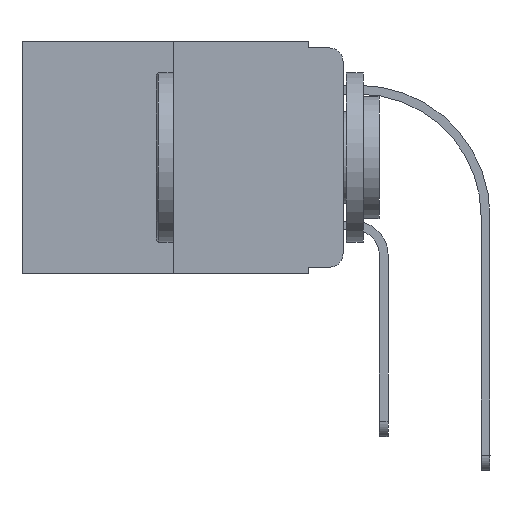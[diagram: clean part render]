
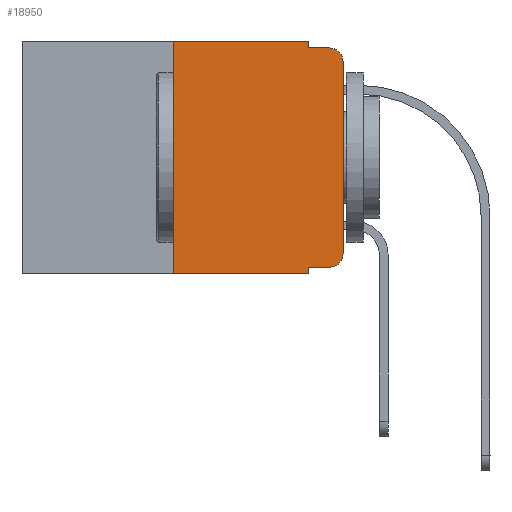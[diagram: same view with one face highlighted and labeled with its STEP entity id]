
A CAD part, left-side view. The second image highlights one B-rep face of the part: STEP entity #18950.
In plain terms, the highlighted planar face has unit normal (-1, 0, 0).
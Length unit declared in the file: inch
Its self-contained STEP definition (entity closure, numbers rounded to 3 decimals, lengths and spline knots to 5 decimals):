
#27 = AXIS2_PLACEMENT_3D ( 'NONE', #23478, #3004, #5293 ) ;
#212 = CARTESIAN_POINT ( 'NONE',  ( 0., 0.02, -0.03 ) ) ;
#581 = VERTEX_POINT ( 'NONE', #647 ) ;
#594 = CIRCLE ( 'NONE', #23664, 0.02 ) ;
#647 = CARTESIAN_POINT ( 'NONE',  ( 0., 0.25, -0.343 ) ) ;
#658 = LINE ( 'NONE', #11733, #10816 ) ;
#1832 = EDGE_CURVE ( 'NONE', #17735, #10853, #594, .T. ) ;
#1859 = ORIENTED_EDGE ( 'NONE', *, *, #13389, .F. ) ;
#2103 = ORIENTED_EDGE ( 'NONE', *, *, #11998, .F. ) ;
#2386 = CARTESIAN_POINT ( 'NONE',  ( 0., 0.051, 0. ) ) ;
#2435 = CARTESIAN_POINT ( 'NONE',  ( 0., 0.02, -0.313 ) ) ;
#2804 = DIRECTION ( 'NONE',  ( 0., -1., 0. ) ) ;
#3004 = DIRECTION ( 'NONE',  ( 1., 0., 0. ) ) ;
#3127 = LINE ( 'NONE', #14115, #8540 ) ;
#4176 = VERTEX_POINT ( 'NONE', #21479 ) ;
#4215 = LINE ( 'NONE', #22547, #14150 ) ;
#4911 = CARTESIAN_POINT ( 'NONE',  ( 0., 0.051, -0.333 ) ) ;
#5267 = CARTESIAN_POINT ( 'NONE',  ( 0., 0.051, -0.333 ) ) ;
#5293 = DIRECTION ( 'NONE',  ( 0., 0., -1. ) ) ;
#5890 = DIRECTION ( 'NONE',  ( 0., 0., -1. ) ) ;
#5921 = DIRECTION ( 'NONE',  ( 0., -1., 0. ) ) ;
#5958 = VERTEX_POINT ( 'NONE', #13751 ) ;
#6118 = ORIENTED_EDGE ( 'NONE', *, *, #1832, .T. ) ;
#7302 = DIRECTION ( 'NONE',  ( 0., 0., -1. ) ) ;
#7472 = ORIENTED_EDGE ( 'NONE', *, *, #21072, .T. ) ;
#7590 = DIRECTION ( 'NONE',  ( 0., 0., 1. ) ) ;
#8540 = VECTOR ( 'NONE', #16400, 39.37008 ) ;
#8892 = VECTOR ( 'NONE', #2804, 39.37008 ) ;
#10391 = EDGE_CURVE ( 'NONE', #581, #14768, #11678, .T. ) ;
#10418 = EDGE_LOOP ( 'NONE', ( #20623, #7472, #2103, #12338, #1859, #22718, #11884, #15980, #13289, #6118 ) ) ;
#10816 = VECTOR ( 'NONE', #17046, 39.37008 ) ;
#10853 = VERTEX_POINT ( 'NONE', #14607 ) ;
#10857 = AXIS2_PLACEMENT_3D ( 'NONE', #212, #20437, #19238 ) ;
#11126 = VERTEX_POINT ( 'NONE', #19862 ) ;
#11250 = CIRCLE ( 'NONE', #10857, 0.02 ) ;
#11678 = LINE ( 'NONE', #22404, #20807 ) ;
#11733 = CARTESIAN_POINT ( 'NONE',  ( 0., 0., 0. ) ) ;
#11884 = ORIENTED_EDGE ( 'NONE', *, *, #20402, .T. ) ;
#11998 = EDGE_CURVE ( 'NONE', #5958, #20988, #12323, .T. ) ;
#12323 = LINE ( 'NONE', #21846, #22447 ) ;
#12338 = ORIENTED_EDGE ( 'NONE', *, *, #15629, .F. ) ;
#12534 = PLANE ( 'NONE',  #27 ) ;
#12624 = DIRECTION ( 'NONE',  ( -1., 0., 0. ) ) ;
#13283 = VERTEX_POINT ( 'NONE', #20157 ) ;
#13289 = ORIENTED_EDGE ( 'NONE', *, *, #19172, .T. ) ;
#13389 = EDGE_CURVE ( 'NONE', #14768, #13283, #4215, .T. ) ;
#13458 = CARTESIAN_POINT ( 'NONE',  ( 0., 0.02, -0.333 ) ) ;
#13751 = CARTESIAN_POINT ( 'NONE',  ( 0., 0.051, -0.01 ) ) ;
#14115 = CARTESIAN_POINT ( 'NONE',  ( 0., 0.051, 0. ) ) ;
#14150 = VECTOR ( 'NONE', #5921, 39.37008 ) ;
#14607 = CARTESIAN_POINT ( 'NONE',  ( 0., 0., -0.313 ) ) ;
#14768 = VERTEX_POINT ( 'NONE', #23671 ) ;
#15044 = LINE ( 'NONE', #5267, #23093 ) ;
#15134 = VECTOR ( 'NONE', #5890, 39.37008 ) ;
#15629 = EDGE_CURVE ( 'NONE', #13283, #5958, #3127, .T. ) ;
#15980 = ORIENTED_EDGE ( 'NONE', *, *, #22397, .F. ) ;
#16064 = LINE ( 'NONE', #23400, #8892 ) ;
#16400 = DIRECTION ( 'NONE',  ( 0., 0., -1. ) ) ;
#17046 = DIRECTION ( 'NONE',  ( 0., 0., 1. ) ) ;
#17735 = VERTEX_POINT ( 'NONE', #13458 ) ;
#18950 = ADVANCED_FACE ( 'NONE', ( #22894 ), #12534, .F. ) ;
#19172 = EDGE_CURVE ( 'NONE', #19557, #17735, #15044, .T. ) ;
#19238 = DIRECTION ( 'NONE',  ( 0., 0., -1. ) ) ;
#19557 = VERTEX_POINT ( 'NONE', #4911 ) ;
#19674 = DIRECTION ( 'NONE',  ( 0., -1., 0. ) ) ;
#19862 = CARTESIAN_POINT ( 'NONE',  ( 0., 0., -0.03 ) ) ;
#20157 = CARTESIAN_POINT ( 'NONE',  ( 0., 0.051, 0. ) ) ;
#20217 = CARTESIAN_POINT ( 'NONE',  ( 0., 0.02, -0.01 ) ) ;
#20229 = EDGE_CURVE ( 'NONE', #10853, #11126, #658, .T. ) ;
#20402 = EDGE_CURVE ( 'NONE', #581, #4176, #16064, .T. ) ;
#20437 = DIRECTION ( 'NONE',  ( -1., 0., 0. ) ) ;
#20623 = ORIENTED_EDGE ( 'NONE', *, *, #20229, .T. ) ;
#20807 = VECTOR ( 'NONE', #7590, 39.37008 ) ;
#20988 = VERTEX_POINT ( 'NONE', #20217 ) ;
#21072 = EDGE_CURVE ( 'NONE', #11126, #20988, #11250, .T. ) ;
#21479 = CARTESIAN_POINT ( 'NONE',  ( 0., 0.051, -0.343 ) ) ;
#21846 = CARTESIAN_POINT ( 'NONE',  ( 0., 0.051, -0.01 ) ) ;
#22391 = DIRECTION ( 'NONE',  ( 0., -1., 0. ) ) ;
#22397 = EDGE_CURVE ( 'NONE', #19557, #4176, #22400, .T. ) ;
#22400 = LINE ( 'NONE', #2386, #15134 ) ;
#22404 = CARTESIAN_POINT ( 'NONE',  ( 0., 0.25, 0. ) ) ;
#22447 = VECTOR ( 'NONE', #19674, 39.37008 ) ;
#22547 = CARTESIAN_POINT ( 'NONE',  ( 0., 0.473, 0. ) ) ;
#22718 = ORIENTED_EDGE ( 'NONE', *, *, #10391, .F. ) ;
#22894 = FACE_OUTER_BOUND ( 'NONE', #10418, .T. ) ;
#23093 = VECTOR ( 'NONE', #22391, 39.37008 ) ;
#23400 = CARTESIAN_POINT ( 'NONE',  ( 0., 0.473, -0.343 ) ) ;
#23478 = CARTESIAN_POINT ( 'NONE',  ( 0., 0.473, 0. ) ) ;
#23664 = AXIS2_PLACEMENT_3D ( 'NONE', #2435, #12624, #7302 ) ;
#23671 = CARTESIAN_POINT ( 'NONE',  ( 0., 0.25, 0. ) ) ;
